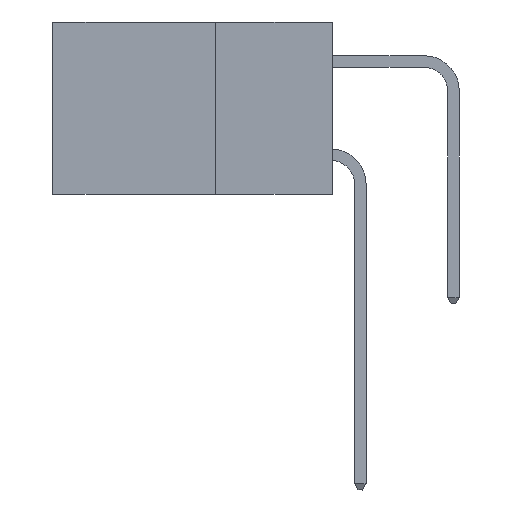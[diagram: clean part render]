
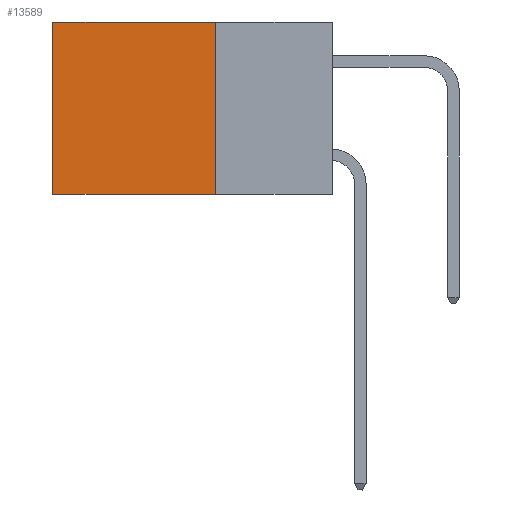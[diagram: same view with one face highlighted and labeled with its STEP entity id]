
A CAD part, left-side view. The second image highlights one B-rep face of the part: STEP entity #13589.
In plain terms, the highlighted planar face has unit normal (-1, 0, 0).
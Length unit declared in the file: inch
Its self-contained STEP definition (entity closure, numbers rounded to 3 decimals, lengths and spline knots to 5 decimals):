
#41 = EDGE_CURVE ( 'NONE', #4110, #11964, #9900, .T. ) ;
#2143 = EDGE_CURVE ( 'NONE', #3767, #16368, #7828, .T. ) ;
#2802 = DIRECTION ( 'NONE',  ( 1., 0., 0. ) ) ;
#3767 = VERTEX_POINT ( 'NONE', #8783 ) ;
#4110 = VERTEX_POINT ( 'NONE', #16471 ) ;
#4638 = DIRECTION ( 'NONE',  ( 0., 1., 0. ) ) ;
#4715 = LINE ( 'NONE', #8016, #14966 ) ;
#4773 = EDGE_CURVE ( 'NONE', #16368, #11964, #4715, .T. ) ;
#5041 = AXIS2_PLACEMENT_3D ( 'NONE', #12741, #2802, #14105 ) ;
#5132 = LINE ( 'NONE', #10535, #9533 ) ;
#6013 = ORIENTED_EDGE ( 'NONE', *, *, #9555, .F. ) ;
#6138 = ORIENTED_EDGE ( 'NONE', *, *, #2143, .T. ) ;
#7828 = LINE ( 'NONE', #15928, #8502 ) ;
#8016 = CARTESIAN_POINT ( 'NONE',  ( 0.298, 0.6, 0. ) ) ;
#8502 = VECTOR ( 'NONE', #10341, 39.37008 ) ;
#8783 = CARTESIAN_POINT ( 'NONE',  ( 0.298, 0.25, 0. ) ) ;
#8975 = FACE_OUTER_BOUND ( 'NONE', #9263, .T. ) ;
#9263 = EDGE_LOOP ( 'NONE', ( #15609, #11055, #6013, #6138 ) ) ;
#9533 = VECTOR ( 'NONE', #15946, 39.37008 ) ;
#9555 = EDGE_CURVE ( 'NONE', #3767, #4110, #5132, .T. ) ;
#9900 = LINE ( 'NONE', #12974, #12927 ) ;
#10341 = DIRECTION ( 'NONE',  ( 0., 1., 0. ) ) ;
#10535 = CARTESIAN_POINT ( 'NONE',  ( 0.298, 0.25, 0. ) ) ;
#11055 = ORIENTED_EDGE ( 'NONE', *, *, #41, .F. ) ;
#11964 = VERTEX_POINT ( 'NONE', #18063 ) ;
#12382 = DIRECTION ( 'NONE',  ( 0., 0., -1. ) ) ;
#12475 = CARTESIAN_POINT ( 'NONE',  ( 0.298, 0.6, 0. ) ) ;
#12496 = PLANE ( 'NONE',  #5041 ) ;
#12741 = CARTESIAN_POINT ( 'NONE',  ( 0.298, 0.25, 0. ) ) ;
#12927 = VECTOR ( 'NONE', #4638, 39.37008 ) ;
#12974 = CARTESIAN_POINT ( 'NONE',  ( 0.298, 0.25, -0.37 ) ) ;
#13589 = ADVANCED_FACE ( 'NONE', ( #8975 ), #12496, .F. ) ;
#14105 = DIRECTION ( 'NONE',  ( 0., 0., -1. ) ) ;
#14966 = VECTOR ( 'NONE', #12382, 39.37008 ) ;
#15609 = ORIENTED_EDGE ( 'NONE', *, *, #4773, .T. ) ;
#15928 = CARTESIAN_POINT ( 'NONE',  ( 0.298, 0.25, 0. ) ) ;
#15946 = DIRECTION ( 'NONE',  ( 0., 0., -1. ) ) ;
#16368 = VERTEX_POINT ( 'NONE', #12475 ) ;
#16471 = CARTESIAN_POINT ( 'NONE',  ( 0.298, 0.25, -0.37 ) ) ;
#18063 = CARTESIAN_POINT ( 'NONE',  ( 0.298, 0.6, -0.37 ) ) ;
